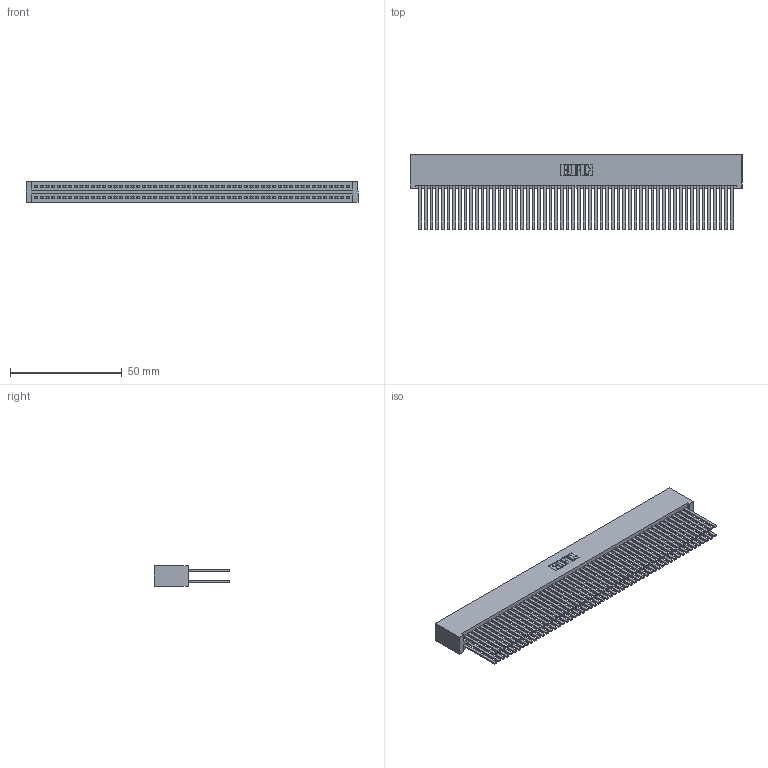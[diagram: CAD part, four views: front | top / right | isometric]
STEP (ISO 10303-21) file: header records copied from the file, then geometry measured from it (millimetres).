
FILE_DESCRIPTION (( 'STEP AP203' ), '1' );
FILE_NAME ('395-112-544-201.STEP', '2019-10-27T15:36:43', ( '' ), ( '' ), 'SwSTEP 2.0', 'SolidWorks 2016', '' );
FILE_SCHEMA (( 'CONFIG_CONTROL_DESIGN' ));
Length unit declared in the file: inch
Products named in the file (3): 395-112-544-201; 345 Part_No Mounting Lugs; 345-292-001_345-293-144
Assembly tree (113 placements, depth 2):
  395-112-544-201
    345 Part_No Mounting Lugs
    345-292-001_345-293-144  x112
Bounding box: 148.84 x 33.96 x 9.4 mm (x, y, z)
Volume: 16774.7 mm3; surface area: 29972 mm2
Topology: 113 solids, 113 shells, 5046 faces, 14989 edges, 9842 vertices
Faces by surface type: plane 3324, cylinder 1722
Entity records: 41593 total; most frequent: CARTESIAN_POINT 6956, ORIENTED_EDGE 6890, DIRECTION 6109, EDGE_CURVE 3445, LINE 3101, VECTOR 3101, VERTEX_POINT 2294, AXIS2_PLACEMENT_3D 1504
